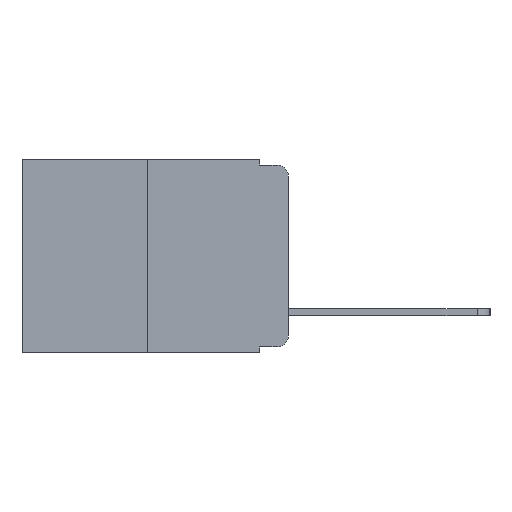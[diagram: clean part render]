
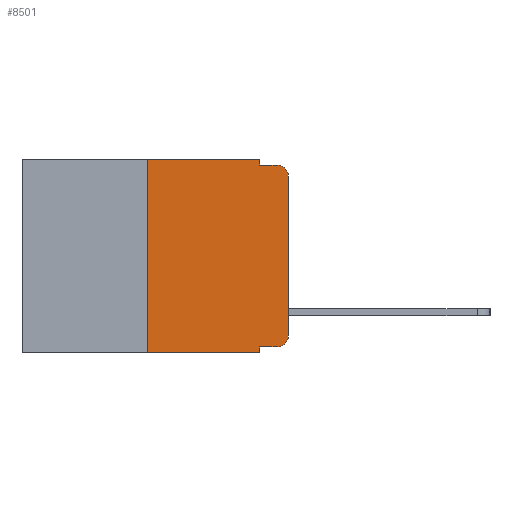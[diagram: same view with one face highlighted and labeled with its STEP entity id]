
A CAD part, left-side view. The second image highlights one B-rep face of the part: STEP entity #8501.
In plain terms, the highlighted planar face has unit normal (-1, 0, 0).
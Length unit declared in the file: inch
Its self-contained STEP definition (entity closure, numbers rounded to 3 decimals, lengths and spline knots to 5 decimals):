
#314 = VECTOR ( 'NONE', #4463, 39.37008 ) ;
#563 = VERTEX_POINT ( 'NONE', #4337 ) ;
#781 = CARTESIAN_POINT ( 'NONE',  ( 0., 0.25, 0. ) ) ;
#795 = LINE ( 'NONE', #6734, #314 ) ;
#1202 = EDGE_LOOP ( 'NONE', ( #13252, #4546, #7546, #1731, #10952, #13976, #11306, #8583, #14688, #5957 ) ) ;
#1256 = VERTEX_POINT ( 'NONE', #10930 ) ;
#1371 = CARTESIAN_POINT ( 'NONE',  ( 0., 0.051, -0.333 ) ) ;
#1423 = EDGE_CURVE ( 'NONE', #5784, #1454, #5288, .T. ) ;
#1454 = VERTEX_POINT ( 'NONE', #5353 ) ;
#1461 = CARTESIAN_POINT ( 'NONE',  ( 0., 0.051, 0. ) ) ;
#1731 = ORIENTED_EDGE ( 'NONE', *, *, #14097, .F. ) ;
#1940 = AXIS2_PLACEMENT_3D ( 'NONE', #10673, #6168, #14108 ) ;
#2270 = EDGE_CURVE ( 'NONE', #6040, #5784, #2580, .T. ) ;
#2419 = CARTESIAN_POINT ( 'NONE',  ( 0., 0.051, -0.343 ) ) ;
#2512 = DIRECTION ( 'NONE',  ( 0., 0., -1. ) ) ;
#2580 = LINE ( 'NONE', #8206, #7955 ) ;
#2624 = VECTOR ( 'NONE', #3616, 39.37008 ) ;
#2658 = LINE ( 'NONE', #1371, #5423 ) ;
#3616 = DIRECTION ( 'NONE',  ( 0., 0., 1. ) ) ;
#3662 = CARTESIAN_POINT ( 'NONE',  ( 0., 0.25, 0. ) ) ;
#4123 = LINE ( 'NONE', #12376, #12840 ) ;
#4337 = CARTESIAN_POINT ( 'NONE',  ( 0., 0.02, -0.333 ) ) ;
#4374 = VECTOR ( 'NONE', #12360, 39.37008 ) ;
#4463 = DIRECTION ( 'NONE',  ( 0., -1., 0. ) ) ;
#4546 = ORIENTED_EDGE ( 'NONE', *, *, #1423, .T. ) ;
#4586 = DIRECTION ( 'NONE',  ( 0., -1., 0. ) ) ;
#4666 = DIRECTION ( 'NONE',  ( 0., 0., -1. ) ) ;
#4846 = CARTESIAN_POINT ( 'NONE',  ( 0., 0.473, 0. ) ) ;
#5059 = EDGE_CURVE ( 'NONE', #13346, #11206, #7017, .T. ) ;
#5288 = CIRCLE ( 'NONE', #1940, 0.02 ) ;
#5353 = CARTESIAN_POINT ( 'NONE',  ( 0., 0.02, -0.01 ) ) ;
#5423 = VECTOR ( 'NONE', #11849, 39.37008 ) ;
#5658 = DIRECTION ( 'NONE',  ( -1., 0., 0. ) ) ;
#5784 = VERTEX_POINT ( 'NONE', #14727 ) ;
#5933 = LINE ( 'NONE', #11398, #14666 ) ;
#5957 = ORIENTED_EDGE ( 'NONE', *, *, #11032, .T. ) ;
#6040 = VERTEX_POINT ( 'NONE', #12961 ) ;
#6064 = LINE ( 'NONE', #11480, #14798 ) ;
#6168 = DIRECTION ( 'NONE',  ( -1., 0., 0. ) ) ;
#6734 = CARTESIAN_POINT ( 'NONE',  ( 0., 0.051, -0.01 ) ) ;
#6756 = VERTEX_POINT ( 'NONE', #11635 ) ;
#7017 = LINE ( 'NONE', #10078, #4374 ) ;
#7107 = DIRECTION ( 'NONE',  ( 0., 0., 1. ) ) ;
#7546 = ORIENTED_EDGE ( 'NONE', *, *, #14860, .F. ) ;
#7824 = AXIS2_PLACEMENT_3D ( 'NONE', #12475, #5658, #13631 ) ;
#7955 = VECTOR ( 'NONE', #7107, 39.37008 ) ;
#8206 = CARTESIAN_POINT ( 'NONE',  ( 0., 0., 0. ) ) ;
#8448 = VERTEX_POINT ( 'NONE', #2419 ) ;
#8501 = ADVANCED_FACE ( 'NONE', ( #13363 ), #15093, .F. ) ;
#8583 = ORIENTED_EDGE ( 'NONE', *, *, #12551, .F. ) ;
#9341 = DIRECTION ( 'NONE',  ( 1., 0., 0. ) ) ;
#9575 = AXIS2_PLACEMENT_3D ( 'NONE', #4846, #9341, #2512 ) ;
#10078 = CARTESIAN_POINT ( 'NONE',  ( 0., 0.473, 0. ) ) ;
#10375 = CARTESIAN_POINT ( 'NONE',  ( 0., 0.051, -0.333 ) ) ;
#10673 = CARTESIAN_POINT ( 'NONE',  ( 0., 0.02, -0.03 ) ) ;
#10930 = CARTESIAN_POINT ( 'NONE',  ( 0., 0.25, -0.343 ) ) ;
#10952 = ORIENTED_EDGE ( 'NONE', *, *, #5059, .F. ) ;
#11032 = EDGE_CURVE ( 'NONE', #563, #6040, #12579, .T. ) ;
#11206 = VERTEX_POINT ( 'NONE', #1461 ) ;
#11228 = DIRECTION ( 'NONE',  ( 0., 0., -1. ) ) ;
#11306 = ORIENTED_EDGE ( 'NONE', *, *, #11988, .T. ) ;
#11398 = CARTESIAN_POINT ( 'NONE',  ( 0., 0.473, -0.343 ) ) ;
#11480 = CARTESIAN_POINT ( 'NONE',  ( 0., 0.051, 0. ) ) ;
#11635 = CARTESIAN_POINT ( 'NONE',  ( 0., 0.051, -0.01 ) ) ;
#11790 = LINE ( 'NONE', #781, #2624 ) ;
#11794 = EDGE_CURVE ( 'NONE', #12686, #563, #2658, .T. ) ;
#11849 = DIRECTION ( 'NONE',  ( 0., -1., 0. ) ) ;
#11988 = EDGE_CURVE ( 'NONE', #1256, #8448, #5933, .T. ) ;
#12360 = DIRECTION ( 'NONE',  ( 0., -1., 0. ) ) ;
#12376 = CARTESIAN_POINT ( 'NONE',  ( 0., 0.051, 0. ) ) ;
#12475 = CARTESIAN_POINT ( 'NONE',  ( 0., 0.02, -0.313 ) ) ;
#12551 = EDGE_CURVE ( 'NONE', #12686, #8448, #4123, .T. ) ;
#12579 = CIRCLE ( 'NONE', #7824, 0.02 ) ;
#12686 = VERTEX_POINT ( 'NONE', #10375 ) ;
#12840 = VECTOR ( 'NONE', #11228, 39.37008 ) ;
#12961 = CARTESIAN_POINT ( 'NONE',  ( 0., 0., -0.313 ) ) ;
#13252 = ORIENTED_EDGE ( 'NONE', *, *, #2270, .T. ) ;
#13314 = EDGE_CURVE ( 'NONE', #1256, #13346, #11790, .T. ) ;
#13346 = VERTEX_POINT ( 'NONE', #3662 ) ;
#13363 = FACE_OUTER_BOUND ( 'NONE', #1202, .T. ) ;
#13631 = DIRECTION ( 'NONE',  ( 0., 0., -1. ) ) ;
#13976 = ORIENTED_EDGE ( 'NONE', *, *, #13314, .F. ) ;
#14097 = EDGE_CURVE ( 'NONE', #11206, #6756, #6064, .T. ) ;
#14108 = DIRECTION ( 'NONE',  ( 0., 0., -1. ) ) ;
#14666 = VECTOR ( 'NONE', #4586, 39.37008 ) ;
#14688 = ORIENTED_EDGE ( 'NONE', *, *, #11794, .T. ) ;
#14727 = CARTESIAN_POINT ( 'NONE',  ( 0., 0., -0.03 ) ) ;
#14798 = VECTOR ( 'NONE', #4666, 39.37008 ) ;
#14860 = EDGE_CURVE ( 'NONE', #6756, #1454, #795, .T. ) ;
#15093 = PLANE ( 'NONE',  #9575 ) ;
